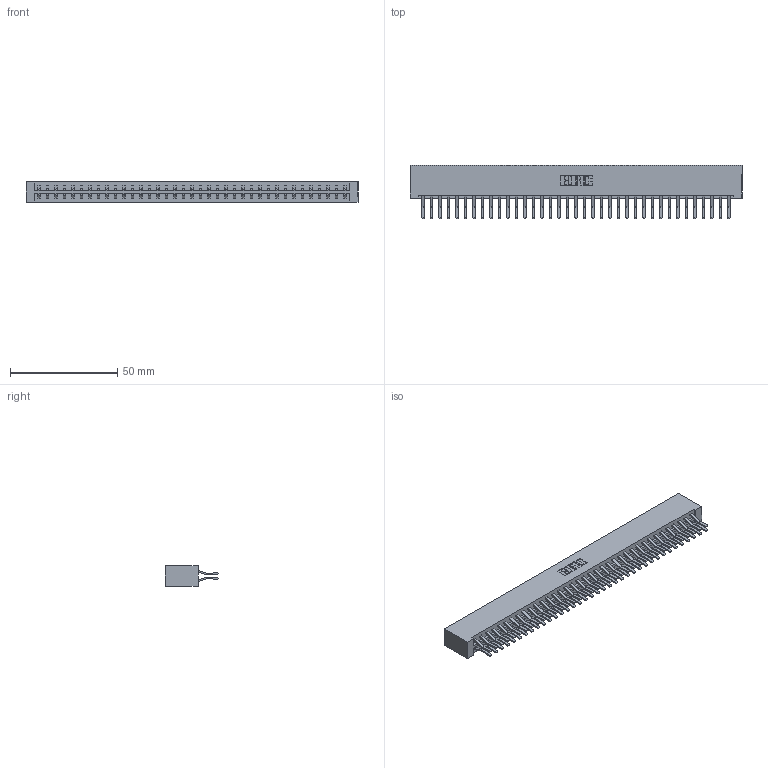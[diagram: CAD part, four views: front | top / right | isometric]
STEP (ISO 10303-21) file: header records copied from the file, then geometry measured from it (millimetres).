
FILE_DESCRIPTION (( 'STEP AP203' ), '1' );
FILE_NAME ('833-074-560-201.STEP', '2020-06-05T17:33:40', ( '' ), ( '' ), 'SwSTEP 2.0', 'SolidWorks 2020', '' );
FILE_SCHEMA (( 'CONFIG_CONTROL_DESIGN' ));
Length unit declared in the file: inch
Products named in the file (3): 833 Part_Lugless; 345-292-001_560 Tail; 833-074-560-201
Assembly tree (75 placements, depth 2):
  833-074-560-201
    833 Part_Lugless
    345-292-001_560 Tail  x74
Bounding box: 154.86 x 24.78 x 9.4 mm (x, y, z)
Volume: 16881.2 mm3; surface area: 21312.1 mm2
Topology: 75 solids, 75 shells, 4102 faces, 12201 edges, 8034 vertices
Faces by surface type: plane 2730, cylinder 1372
Entity records: 24261 total; most frequent: CARTESIAN_POINT 4026, ORIENTED_EDGE 3962, DIRECTION 3445, EDGE_CURVE 1981, VECTOR 1857, LINE 1857, VERTEX_POINT 1318, AXIS2_PLACEMENT_3D 794
